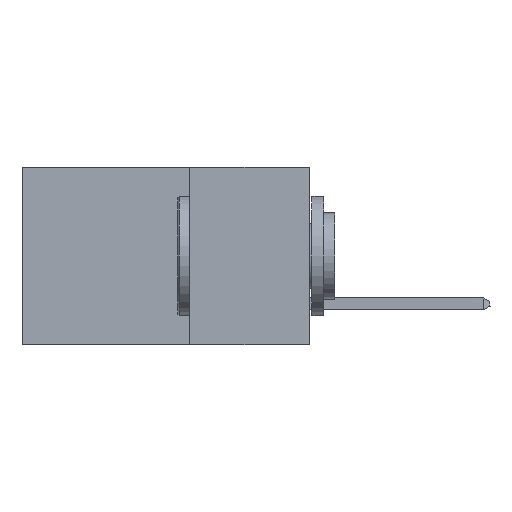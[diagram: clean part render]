
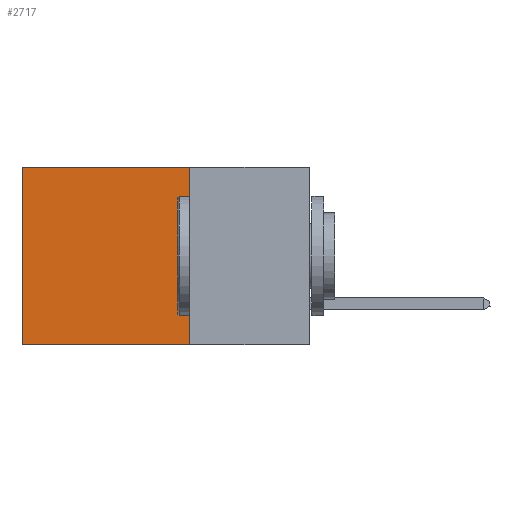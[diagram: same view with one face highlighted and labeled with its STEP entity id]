
A CAD part, left-side view. The second image highlights one B-rep face of the part: STEP entity #2717.
In plain terms, the highlighted planar face has unit normal (-1, 0, 0).
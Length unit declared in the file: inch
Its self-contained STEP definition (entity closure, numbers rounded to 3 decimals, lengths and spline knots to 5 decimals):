
#110 = CARTESIAN_POINT ( 'NONE',  ( 0.2875, 0.25, 0. ) ) ;
#810 = DIRECTION ( 'NONE',  ( 1., 0., 0. ) ) ;
#1492 = ORIENTED_EDGE ( 'NONE', *, *, #6597, .F. ) ;
#1787 = LINE ( 'NONE', #9188, #4961 ) ;
#2034 = ORIENTED_EDGE ( 'NONE', *, *, #5667, .T. ) ;
#2717 = ADVANCED_FACE ( 'NONE', ( #9434 ), #10190, .F. ) ;
#3763 = CARTESIAN_POINT ( 'NONE',  ( 0.2875, 0.25, 0. ) ) ;
#4760 = DIRECTION ( 'NONE',  ( 0., 1., 0. ) ) ;
#4961 = VECTOR ( 'NONE', #10535, 39.37008 ) ;
#5667 = EDGE_CURVE ( 'NONE', #11678, #17061, #9324, .T. ) ;
#5680 = CARTESIAN_POINT ( 'NONE',  ( 0.2875, 0.6, 0. ) ) ;
#5749 = VECTOR ( 'NONE', #16427, 39.37008 ) ;
#5792 = ORIENTED_EDGE ( 'NONE', *, *, #11265, .T. ) ;
#5808 = CARTESIAN_POINT ( 'NONE',  ( 0.2875, 0.6, 0. ) ) ;
#6221 = CARTESIAN_POINT ( 'NONE',  ( 0.2875, 0.25, -0.37 ) ) ;
#6346 = LINE ( 'NONE', #3763, #10113 ) ;
#6597 = EDGE_CURVE ( 'NONE', #9781, #7807, #13742, .T. ) ;
#7807 = VERTEX_POINT ( 'NONE', #6221 ) ;
#9188 = CARTESIAN_POINT ( 'NONE',  ( 0.2875, 0.25, -0.37 ) ) ;
#9212 = CARTESIAN_POINT ( 'NONE',  ( 0.2875, 0.25, 0. ) ) ;
#9324 = LINE ( 'NONE', #5680, #5749 ) ;
#9350 = AXIS2_PLACEMENT_3D ( 'NONE', #16771, #810, #12880 ) ;
#9434 = FACE_OUTER_BOUND ( 'NONE', #16107, .T. ) ;
#9781 = VERTEX_POINT ( 'NONE', #110 ) ;
#10113 = VECTOR ( 'NONE', #4760, 39.37008 ) ;
#10190 = PLANE ( 'NONE',  #9350 ) ;
#10535 = DIRECTION ( 'NONE',  ( 0., 1., 0. ) ) ;
#11265 = EDGE_CURVE ( 'NONE', #9781, #11678, #6346, .T. ) ;
#11496 = CARTESIAN_POINT ( 'NONE',  ( 0.2875, 0.6, -0.37 ) ) ;
#11678 = VERTEX_POINT ( 'NONE', #5808 ) ;
#12880 = DIRECTION ( 'NONE',  ( 0., 0., -1. ) ) ;
#13263 = DIRECTION ( 'NONE',  ( 0., 0., -1. ) ) ;
#13742 = LINE ( 'NONE', #9212, #16452 ) ;
#14368 = EDGE_CURVE ( 'NONE', #7807, #17061, #1787, .T. ) ;
#16107 = EDGE_LOOP ( 'NONE', ( #2034, #16536, #1492, #5792 ) ) ;
#16427 = DIRECTION ( 'NONE',  ( 0., 0., -1. ) ) ;
#16452 = VECTOR ( 'NONE', #13263, 39.37008 ) ;
#16536 = ORIENTED_EDGE ( 'NONE', *, *, #14368, .F. ) ;
#16771 = CARTESIAN_POINT ( 'NONE',  ( 0.2875, 0.25, 0. ) ) ;
#17061 = VERTEX_POINT ( 'NONE', #11496 ) ;
